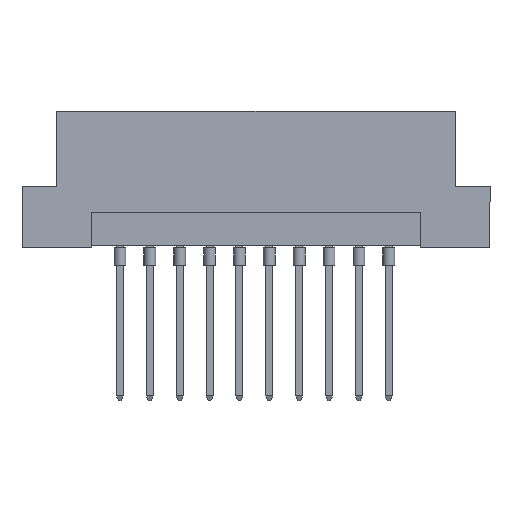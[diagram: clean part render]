
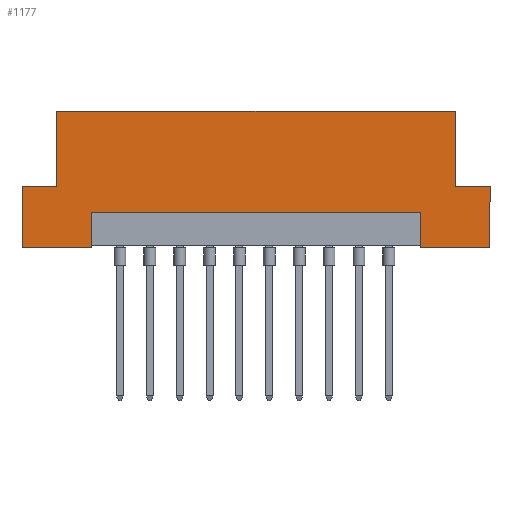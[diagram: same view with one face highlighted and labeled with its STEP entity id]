
A CAD part, front view. The second image highlights one B-rep face of the part: STEP entity #1177.
In plain terms, the highlighted planar face has unit normal (0, -1, 0).
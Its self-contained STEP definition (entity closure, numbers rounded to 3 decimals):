
#70 = EDGE_CURVE ( 'NONE', #301, #4235, #3606, .T. ) ;
#296 = VERTEX_POINT ( 'NONE', #1690 ) ;
#301 = VERTEX_POINT ( 'NONE', #3444 ) ;
#332 = DIRECTION ( 'NONE',  ( 1., 0., 0. ) ) ;
#404 = VECTOR ( 'NONE', #4338, 1000. ) ;
#448 = EDGE_CURVE ( 'NONE', #4278, #2378, #3677, .T. ) ;
#459 = DIRECTION ( 'NONE',  ( 0., 0., 1. ) ) ;
#849 = LINE ( 'NONE', #1181, #3644 ) ;
#880 = EDGE_CURVE ( 'NONE', #2378, #5635, #3899, .T. ) ;
#927 = EDGE_CURVE ( 'NONE', #1139, #296, #5211, .T. ) ;
#964 = EDGE_CURVE ( 'NONE', #4486, #301, #849, .T. ) ;
#1079 = EDGE_CURVE ( 'NONE', #4278, #4044, #1954, .T. ) ;
#1121 = CARTESIAN_POINT ( 'NONE',  ( -14., -4.3, 0. ) ) ;
#1139 = VERTEX_POINT ( 'NONE', #2955 ) ;
#1177 = ADVANCED_FACE ( 'NONE', ( #5569 ), #2044, .F. ) ;
#1181 = CARTESIAN_POINT ( 'NONE',  ( 19.9, -4.3, 5.2 ) ) ;
#1238 = EDGE_CURVE ( 'NONE', #4486, #296, #5341, .T. ) ;
#1246 = CARTESIAN_POINT ( 'NONE',  ( 14., -4.3, 0. ) ) ;
#1248 = DIRECTION ( 'NONE',  ( 0., 1., 0. ) ) ;
#1267 = ORIENTED_EDGE ( 'NONE', *, *, #2948, .F. ) ;
#1282 = CARTESIAN_POINT ( 'NONE',  ( 19.9, -4.3, 11.6 ) ) ;
#1338 = EDGE_LOOP ( 'NONE', ( #3000, #1267, #4448, #2448, #4550, #4251, #5482, #3269, #2176, #2713, #2711, #3836 ) ) ;
#1378 = DIRECTION ( 'NONE',  ( 0., 0., 1. ) ) ;
#1563 = CARTESIAN_POINT ( 'NONE',  ( -16.94, -4.3, 5.2 ) ) ;
#1592 = CARTESIAN_POINT ( 'NONE',  ( 19.9, -4.3, 0. ) ) ;
#1690 = CARTESIAN_POINT ( 'NONE',  ( 16.94, -4.3, 11.6 ) ) ;
#1926 = CARTESIAN_POINT ( 'NONE',  ( 16.94, -4.3, 5.2 ) ) ;
#1930 = DIRECTION ( 'NONE',  ( 1., 0., 0. ) ) ;
#1954 = LINE ( 'NONE', #4644, #5189 ) ;
#2020 = VERTEX_POINT ( 'NONE', #1246 ) ;
#2044 = PLANE ( 'NONE',  #2528 ) ;
#2127 = LINE ( 'NONE', #2211, #404 ) ;
#2175 = VECTOR ( 'NONE', #332, 1000. ) ;
#2176 = ORIENTED_EDGE ( 'NONE', *, *, #1079, .F. ) ;
#2211 = CARTESIAN_POINT ( 'NONE',  ( -14., -4.3, 0.2 ) ) ;
#2219 = LINE ( 'NONE', #3067, #5471 ) ;
#2295 = DIRECTION ( 'NONE',  ( 1., 0., 0. ) ) ;
#2314 = CARTESIAN_POINT ( 'NONE',  ( -19.9, -4.3, 0. ) ) ;
#2328 = CARTESIAN_POINT ( 'NONE',  ( -14., -4.3, 3. ) ) ;
#2378 = VERTEX_POINT ( 'NONE', #2314 ) ;
#2448 = ORIENTED_EDGE ( 'NONE', *, *, #70, .F. ) ;
#2451 = VECTOR ( 'NONE', #5559, 1000. ) ;
#2512 = LINE ( 'NONE', #3824, #2451 ) ;
#2528 = AXIS2_PLACEMENT_3D ( 'NONE', #4269, #1248, #3393 ) ;
#2711 = ORIENTED_EDGE ( 'NONE', *, *, #880, .T. ) ;
#2713 = ORIENTED_EDGE ( 'NONE', *, *, #448, .T. ) ;
#2865 = CARTESIAN_POINT ( 'NONE',  ( 14., -4.3, 3. ) ) ;
#2917 = DIRECTION ( 'NONE',  ( 1., 0., 0. ) ) ;
#2948 = EDGE_CURVE ( 'NONE', #2020, #5102, #4103, .T. ) ;
#2955 = CARTESIAN_POINT ( 'NONE',  ( -16.94, -4.3, 11.6 ) ) ;
#3000 = ORIENTED_EDGE ( 'NONE', *, *, #3884, .T. ) ;
#3067 = CARTESIAN_POINT ( 'NONE',  ( -16.94, -4.3, 5.2 ) ) ;
#3241 = VECTOR ( 'NONE', #4931, 1000. ) ;
#3269 = ORIENTED_EDGE ( 'NONE', *, *, #4826, .F. ) ;
#3272 = VECTOR ( 'NONE', #459, 1000. ) ;
#3393 = DIRECTION ( 'NONE',  ( -1., 0., 0. ) ) ;
#3444 = CARTESIAN_POINT ( 'NONE',  ( 19.9, -4.3, 5.2 ) ) ;
#3589 = LINE ( 'NONE', #4997, #3719 ) ;
#3606 = LINE ( 'NONE', #5343, #5549 ) ;
#3644 = VECTOR ( 'NONE', #2917, 1000. ) ;
#3677 = LINE ( 'NONE', #4065, #3826 ) ;
#3719 = VECTOR ( 'NONE', #2295, 1000. ) ;
#3776 = EDGE_CURVE ( 'NONE', #5117, #5635, #2127, .T. ) ;
#3819 = DIRECTION ( 'NONE',  ( 1., 0., 0. ) ) ;
#3824 = CARTESIAN_POINT ( 'NONE',  ( 19.9, -4.3, 0. ) ) ;
#3826 = VECTOR ( 'NONE', #4534, 1000. ) ;
#3836 = ORIENTED_EDGE ( 'NONE', *, *, #3776, .F. ) ;
#3884 = EDGE_CURVE ( 'NONE', #5117, #5102, #3589, .T. ) ;
#3899 = LINE ( 'NONE', #4742, #4629 ) ;
#3996 = CARTESIAN_POINT ( 'NONE',  ( 16.94, -4.3, 5.2 ) ) ;
#4044 = VERTEX_POINT ( 'NONE', #1563 ) ;
#4053 = CARTESIAN_POINT ( 'NONE',  ( 14., -4.3, 0.2 ) ) ;
#4065 = CARTESIAN_POINT ( 'NONE',  ( -19.9, -4.3, 11.6 ) ) ;
#4103 = LINE ( 'NONE', #4053, #3241 ) ;
#4235 = VERTEX_POINT ( 'NONE', #1592 ) ;
#4251 = ORIENTED_EDGE ( 'NONE', *, *, #1238, .T. ) ;
#4269 = CARTESIAN_POINT ( 'NONE',  ( 19.9, -4.3, 11.6 ) ) ;
#4278 = VERTEX_POINT ( 'NONE', #4786 ) ;
#4338 = DIRECTION ( 'NONE',  ( 0., 0., -1. ) ) ;
#4448 = ORIENTED_EDGE ( 'NONE', *, *, #5159, .T. ) ;
#4486 = VERTEX_POINT ( 'NONE', #1926 ) ;
#4534 = DIRECTION ( 'NONE',  ( 0., 0., -1. ) ) ;
#4550 = ORIENTED_EDGE ( 'NONE', *, *, #964, .F. ) ;
#4629 = VECTOR ( 'NONE', #3819, 1000. ) ;
#4644 = CARTESIAN_POINT ( 'NONE',  ( -19.9, -4.3, 5.2 ) ) ;
#4742 = CARTESIAN_POINT ( 'NONE',  ( 19.9, -4.3, 0. ) ) ;
#4786 = CARTESIAN_POINT ( 'NONE',  ( -19.9, -4.3, 5.2 ) ) ;
#4826 = EDGE_CURVE ( 'NONE', #4044, #1139, #2219, .T. ) ;
#4901 = DIRECTION ( 'NONE',  ( 0., 0., -1. ) ) ;
#4931 = DIRECTION ( 'NONE',  ( 0., 0., 1. ) ) ;
#4997 = CARTESIAN_POINT ( 'NONE',  ( -14., -4.3, 3. ) ) ;
#5102 = VERTEX_POINT ( 'NONE', #2865 ) ;
#5117 = VERTEX_POINT ( 'NONE', #2328 ) ;
#5159 = EDGE_CURVE ( 'NONE', #2020, #4235, #2512, .T. ) ;
#5189 = VECTOR ( 'NONE', #1930, 1000. ) ;
#5211 = LINE ( 'NONE', #1282, #2175 ) ;
#5341 = LINE ( 'NONE', #3996, #3272 ) ;
#5343 = CARTESIAN_POINT ( 'NONE',  ( 19.9, -4.3, 11.6 ) ) ;
#5471 = VECTOR ( 'NONE', #1378, 1000. ) ;
#5482 = ORIENTED_EDGE ( 'NONE', *, *, #927, .F. ) ;
#5549 = VECTOR ( 'NONE', #4901, 1000. ) ;
#5559 = DIRECTION ( 'NONE',  ( 1., 0., 0. ) ) ;
#5569 = FACE_OUTER_BOUND ( 'NONE', #1338, .T. ) ;
#5635 = VERTEX_POINT ( 'NONE', #1121 ) ;
